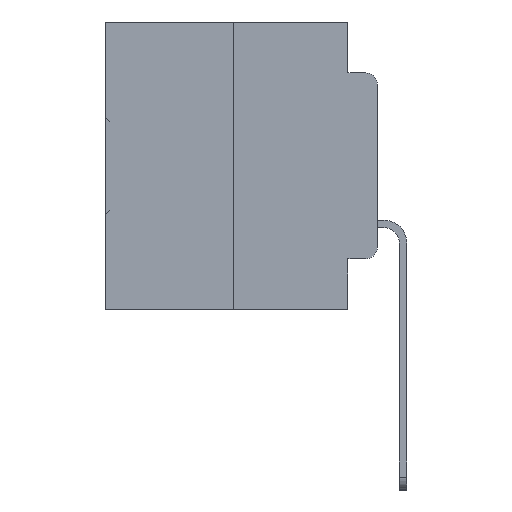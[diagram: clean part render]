
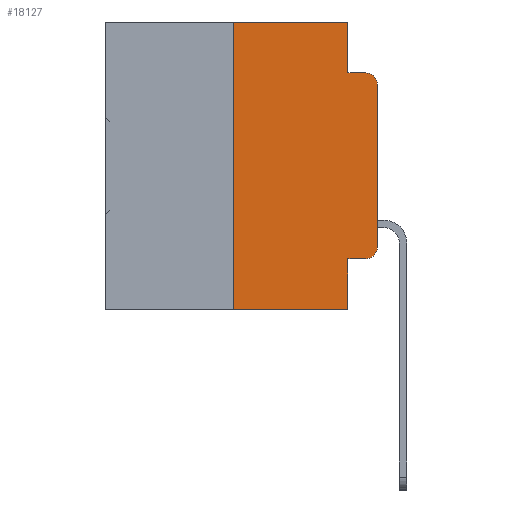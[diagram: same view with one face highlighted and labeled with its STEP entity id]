
A CAD part, left-side view. The second image highlights one B-rep face of the part: STEP entity #18127.
In plain terms, the highlighted planar face has unit normal (-1, 0, 0).
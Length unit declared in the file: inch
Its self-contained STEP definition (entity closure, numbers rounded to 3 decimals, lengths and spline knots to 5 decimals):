
#824 = VECTOR ( 'NONE', #33970, 39.37008 ) ;
#838 = CARTESIAN_POINT ( 'NONE',  ( 0., 0.051, 0. ) ) ;
#2327 = CARTESIAN_POINT ( 'NONE',  ( 0., 0.473, 0. ) ) ;
#2699 = VECTOR ( 'NONE', #19485, 39.37008 ) ;
#2996 = DIRECTION ( 'NONE',  ( 0., -1., 0. ) ) ;
#3050 = AXIS2_PLACEMENT_3D ( 'NONE', #2327, #10547, #29414 ) ;
#3262 = LINE ( 'NONE', #15534, #30356 ) ;
#3435 = ORIENTED_EDGE ( 'NONE', *, *, #18192, .T. ) ;
#3944 = CARTESIAN_POINT ( 'NONE',  ( 0., 0.051, -0.0885 ) ) ;
#4738 = EDGE_CURVE ( 'NONE', #26437, #6949, #34295, .T. ) ;
#5190 = ORIENTED_EDGE ( 'NONE', *, *, #13658, .F. ) ;
#5219 = EDGE_CURVE ( 'NONE', #28679, #28165, #26023, .T. ) ;
#5386 = DIRECTION ( 'NONE',  ( -1., 0., 0. ) ) ;
#6100 = ORIENTED_EDGE ( 'NONE', *, *, #19480, .T. ) ;
#6949 = VERTEX_POINT ( 'NONE', #30142 ) ;
#7032 = LINE ( 'NONE', #29381, #8734 ) ;
#7129 = VERTEX_POINT ( 'NONE', #17441 ) ;
#7707 = VERTEX_POINT ( 'NONE', #20228 ) ;
#8068 = LINE ( 'NONE', #17959, #824 ) ;
#8098 = LINE ( 'NONE', #25539, #34179 ) ;
#8167 = DIRECTION ( 'NONE',  ( 0., 0., 1. ) ) ;
#8350 = CARTESIAN_POINT ( 'NONE',  ( 0., 0.473, -0.5 ) ) ;
#8663 = ORIENTED_EDGE ( 'NONE', *, *, #22253, .F. ) ;
#8734 = VECTOR ( 'NONE', #32052, 39.37008 ) ;
#10100 = DIRECTION ( 'NONE',  ( 0., 0., -1. ) ) ;
#10309 = ORIENTED_EDGE ( 'NONE', *, *, #19326, .F. ) ;
#10387 = AXIS2_PLACEMENT_3D ( 'NONE', #21657, #5386, #24381 ) ;
#10390 = VERTEX_POINT ( 'NONE', #15444 ) ;
#10547 = DIRECTION ( 'NONE',  ( 1., 0., 0. ) ) ;
#11299 = CARTESIAN_POINT ( 'NONE',  ( 0., 0.25, 0. ) ) ;
#11374 = EDGE_CURVE ( 'NONE', #10390, #7707, #17158, .T. ) ;
#11841 = DIRECTION ( 'NONE',  ( -1., 0., 0. ) ) ;
#12754 = FACE_OUTER_BOUND ( 'NONE', #15686, .T. ) ;
#13658 = EDGE_CURVE ( 'NONE', #7707, #32992, #8068, .T. ) ;
#14527 = EDGE_CURVE ( 'NONE', #28165, #17458, #19629, .T. ) ;
#15444 = CARTESIAN_POINT ( 'NONE',  ( 0., 0.25, -0.5 ) ) ;
#15534 = CARTESIAN_POINT ( 'NONE',  ( 0., 0.051, 0. ) ) ;
#15686 = EDGE_LOOP ( 'NONE', ( #31403, #3435, #18780, #10309, #5190, #20074, #6100, #8663, #28973, #30649 ) ) ;
#16679 = CARTESIAN_POINT ( 'NONE',  ( 0., 0., -0.1085 ) ) ;
#17158 = LINE ( 'NONE', #11299, #2699 ) ;
#17352 = DIRECTION ( 'NONE',  ( 0., -1., 0. ) ) ;
#17441 = CARTESIAN_POINT ( 'NONE',  ( 0., 0.051, -0.4115 ) ) ;
#17458 = VERTEX_POINT ( 'NONE', #16679 ) ;
#17959 = CARTESIAN_POINT ( 'NONE',  ( 0., 0.473, 0. ) ) ;
#18127 = ADVANCED_FACE ( 'NONE', ( #12754 ), #26711, .F. ) ;
#18156 = VECTOR ( 'NONE', #2996, 39.37008 ) ;
#18192 = EDGE_CURVE ( 'NONE', #17458, #6949, #18260, .T. ) ;
#18260 = CIRCLE ( 'NONE', #10387, 0.02 ) ;
#18780 = ORIENTED_EDGE ( 'NONE', *, *, #4738, .F. ) ;
#19326 = EDGE_CURVE ( 'NONE', #32992, #26437, #3262, .T. ) ;
#19480 = EDGE_CURVE ( 'NONE', #10390, #27057, #33235, .T. ) ;
#19485 = DIRECTION ( 'NONE',  ( 0., 0., 1. ) ) ;
#19629 = LINE ( 'NONE', #21680, #33023 ) ;
#20064 = CARTESIAN_POINT ( 'NONE',  ( 0., 0.051, -0.0885 ) ) ;
#20074 = ORIENTED_EDGE ( 'NONE', *, *, #11374, .F. ) ;
#20082 = VECTOR ( 'NONE', #17352, 39.37008 ) ;
#20228 = CARTESIAN_POINT ( 'NONE',  ( 0., 0.25, 0. ) ) ;
#21657 = CARTESIAN_POINT ( 'NONE',  ( 0., 0.02, -0.1085 ) ) ;
#21680 = CARTESIAN_POINT ( 'NONE',  ( 0., 0., 0. ) ) ;
#22253 = EDGE_CURVE ( 'NONE', #7129, #27057, #7032, .T. ) ;
#24381 = DIRECTION ( 'NONE',  ( 0., 0., -1. ) ) ;
#24664 = CARTESIAN_POINT ( 'NONE',  ( 0., 0.02, -0.4115 ) ) ;
#25539 = CARTESIAN_POINT ( 'NONE',  ( 0., 0.051, -0.4115 ) ) ;
#26023 = CIRCLE ( 'NONE', #30582, 0.02 ) ;
#26437 = VERTEX_POINT ( 'NONE', #3944 ) ;
#26711 = PLANE ( 'NONE',  #3050 ) ;
#27057 = VERTEX_POINT ( 'NONE', #30831 ) ;
#28017 = CARTESIAN_POINT ( 'NONE',  ( 0., 0.02, -0.3915 ) ) ;
#28060 = CARTESIAN_POINT ( 'NONE',  ( 0., 0., -0.3915 ) ) ;
#28165 = VERTEX_POINT ( 'NONE', #28060 ) ;
#28219 = DIRECTION ( 'NONE',  ( 0., -1., 0. ) ) ;
#28679 = VERTEX_POINT ( 'NONE', #24664 ) ;
#28973 = ORIENTED_EDGE ( 'NONE', *, *, #29470, .T. ) ;
#29381 = CARTESIAN_POINT ( 'NONE',  ( 0., 0.051, 0. ) ) ;
#29414 = DIRECTION ( 'NONE',  ( 0., 0., -1. ) ) ;
#29470 = EDGE_CURVE ( 'NONE', #7129, #28679, #8098, .T. ) ;
#30142 = CARTESIAN_POINT ( 'NONE',  ( 0., 0.02, -0.0885 ) ) ;
#30356 = VECTOR ( 'NONE', #10100, 39.37008 ) ;
#30582 = AXIS2_PLACEMENT_3D ( 'NONE', #28017, #11841, #30712 ) ;
#30649 = ORIENTED_EDGE ( 'NONE', *, *, #5219, .T. ) ;
#30712 = DIRECTION ( 'NONE',  ( 0., 0., -1. ) ) ;
#30831 = CARTESIAN_POINT ( 'NONE',  ( 0., 0.051, -0.5 ) ) ;
#31403 = ORIENTED_EDGE ( 'NONE', *, *, #14527, .T. ) ;
#32052 = DIRECTION ( 'NONE',  ( 0., 0., -1. ) ) ;
#32992 = VERTEX_POINT ( 'NONE', #838 ) ;
#33023 = VECTOR ( 'NONE', #8167, 39.37008 ) ;
#33235 = LINE ( 'NONE', #8350, #18156 ) ;
#33970 = DIRECTION ( 'NONE',  ( 0., -1., 0. ) ) ;
#34179 = VECTOR ( 'NONE', #28219, 39.37008 ) ;
#34295 = LINE ( 'NONE', #20064, #20082 ) ;
